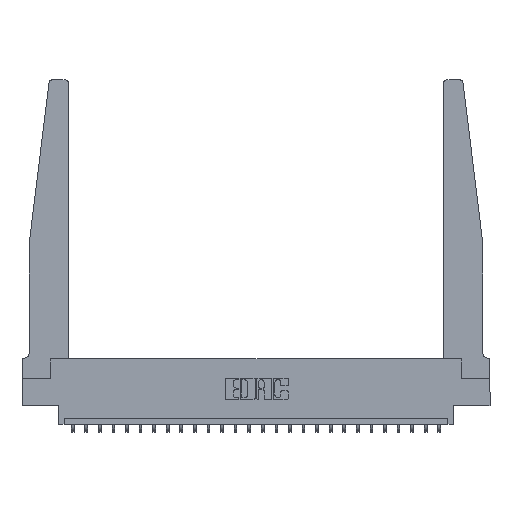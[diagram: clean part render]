
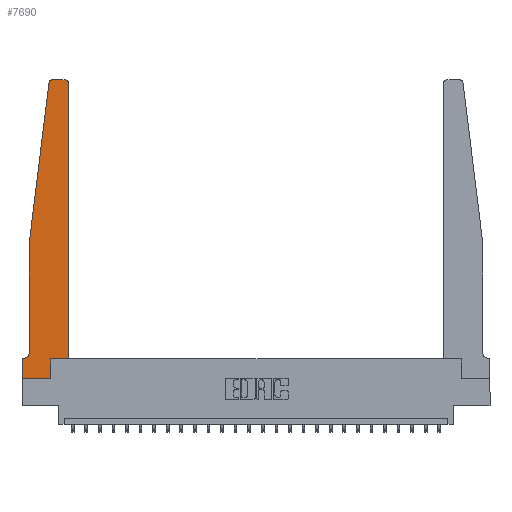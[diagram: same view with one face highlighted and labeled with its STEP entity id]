
A CAD part, top view. The second image highlights one B-rep face of the part: STEP entity #7690.
In plain terms, the highlighted planar face has unit normal (0, 0, 1).
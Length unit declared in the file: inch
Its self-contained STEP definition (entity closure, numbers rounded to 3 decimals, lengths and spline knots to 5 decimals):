
#848 = CIRCLE ( 'NONE', #6700, 0.03 ) ;
#877 = DIRECTION ( 'NONE',  ( 0., -1., 0. ) ) ;
#1224 = CARTESIAN_POINT ( 'NONE',  ( 0.065, 0.2375, 0.37 ) ) ;
#1806 = DIRECTION ( 'NONE',  ( 1., 0., 0. ) ) ;
#1873 = VERTEX_POINT ( 'NONE', #12678 ) ;
#2963 = ORIENTED_EDGE ( 'NONE', *, *, #17596, .T. ) ;
#3009 = VECTOR ( 'NONE', #11508, 39.37008 ) ;
#3305 = EDGE_CURVE ( 'NONE', #21241, #8858, #13547, .T. ) ;
#3498 = LINE ( 'NONE', #13590, #21638 ) ;
#3528 = CARTESIAN_POINT ( 'NONE',  ( 0.395, 2.72, 0.37 ) ) ;
#3732 = CARTESIAN_POINT ( 'NONE',  ( 0.065, 0.1875, 0.37 ) ) ;
#4224 = DIRECTION ( 'NONE',  ( -0.122, -0.992, 0. ) ) ;
#4286 = CARTESIAN_POINT ( 'NONE',  ( 0.2605, 0., 0.37 ) ) ;
#4564 = EDGE_CURVE ( 'NONE', #17738, #1873, #848, .T. ) ;
#4660 = VERTEX_POINT ( 'NONE', #21850 ) ;
#4731 = EDGE_CURVE ( 'NONE', #16725, #4660, #22803, .T. ) ;
#5137 = LINE ( 'NONE', #17966, #23874 ) ;
#5405 = DIRECTION ( 'NONE',  ( 1., 0., 0. ) ) ;
#5540 = VERTEX_POINT ( 'NONE', #5932 ) ;
#5932 = CARTESIAN_POINT ( 'NONE',  ( 0.395, 2.75, 0.37 ) ) ;
#5989 = VERTEX_POINT ( 'NONE', #16567 ) ;
#6015 = CARTESIAN_POINT ( 'NONE',  ( 0., 0., 0.37 ) ) ;
#6136 = DIRECTION ( 'NONE',  ( 1., 0., 0. ) ) ;
#6283 = ORIENTED_EDGE ( 'NONE', *, *, #21321, .T. ) ;
#6534 = VECTOR ( 'NONE', #1806, 39.37008 ) ;
#6631 = CARTESIAN_POINT ( 'NONE',  ( 0.27653, 2.75, 0.37 ) ) ;
#6700 = AXIS2_PLACEMENT_3D ( 'NONE', #10417, #23488, #12304 ) ;
#6841 = EDGE_CURVE ( 'NONE', #10985, #21241, #22988, .T. ) ;
#6980 = EDGE_CURVE ( 'NONE', #5540, #17738, #5137, .T. ) ;
#7046 = EDGE_LOOP ( 'NONE', ( #7578, #17709, #7866, #20436, #24205, #12894, #13224, #21968, #2963, #16415, #7968, #6283 ) ) ;
#7367 = CARTESIAN_POINT ( 'NONE',  ( 0.2605, 0.18, 0.37 ) ) ;
#7578 = ORIENTED_EDGE ( 'NONE', *, *, #6980, .T. ) ;
#7690 = ADVANCED_FACE ( 'NONE', ( #17716 ), #15469, .T. ) ;
#7740 = CARTESIAN_POINT ( 'NONE',  ( 0., 0., 0.37 ) ) ;
#7866 = ORIENTED_EDGE ( 'NONE', *, *, #9949, .T. ) ;
#7924 = DIRECTION ( 'NONE',  ( 1., 0., 0. ) ) ;
#7968 = ORIENTED_EDGE ( 'NONE', *, *, #4731, .T. ) ;
#8472 = LINE ( 'NONE', #6015, #17218 ) ;
#8858 = VERTEX_POINT ( 'NONE', #15163 ) ;
#9049 = CARTESIAN_POINT ( 'NONE',  ( 0.425, 0.18, 0.37 ) ) ;
#9165 = CIRCLE ( 'NONE', #15791, 0.03 ) ;
#9415 = VECTOR ( 'NONE', #11869, 39.37008 ) ;
#9768 = EDGE_CURVE ( 'NONE', #8858, #17679, #10851, .T. ) ;
#9903 = DIRECTION ( 'NONE',  ( 0., 0., -1. ) ) ;
#9949 = EDGE_CURVE ( 'NONE', #1873, #10985, #3498, .T. ) ;
#10417 = CARTESIAN_POINT ( 'NONE',  ( 0.27653, 2.72, 0.37 ) ) ;
#10851 = LINE ( 'NONE', #3732, #15813 ) ;
#10917 = CARTESIAN_POINT ( 'NONE',  ( 0.425, 0.18, 0.37 ) ) ;
#10985 = VERTEX_POINT ( 'NONE', #12646 ) ;
#11508 = DIRECTION ( 'NONE',  ( 0., -1., 0. ) ) ;
#11869 = DIRECTION ( 'NONE',  ( 0., 1., 0. ) ) ;
#12304 = DIRECTION ( 'NONE',  ( 1., 0., 0. ) ) ;
#12646 = CARTESIAN_POINT ( 'NONE',  ( 0.065, 1.25, 0.37 ) ) ;
#12678 = CARTESIAN_POINT ( 'NONE',  ( 0.24675, 2.72367, 0.37 ) ) ;
#12894 = ORIENTED_EDGE ( 'NONE', *, *, #9768, .T. ) ;
#13064 = CARTESIAN_POINT ( 'NONE',  ( 0.425, 0.18, 0.37 ) ) ;
#13224 = ORIENTED_EDGE ( 'NONE', *, *, #20869, .T. ) ;
#13547 = CIRCLE ( 'NONE', #21059, 0.05 ) ;
#13590 = CARTESIAN_POINT ( 'NONE',  ( 0.065, 1.25, 0.37 ) ) ;
#13686 = VERTEX_POINT ( 'NONE', #4286 ) ;
#13914 = CARTESIAN_POINT ( 'NONE',  ( 0., 0.1875, 0.37 ) ) ;
#13995 = CARTESIAN_POINT ( 'NONE',  ( 0.065, 1.25, 0.37 ) ) ;
#14399 = LINE ( 'NONE', #23038, #9415 ) ;
#14655 = VERTEX_POINT ( 'NONE', #7367 ) ;
#15163 = CARTESIAN_POINT ( 'NONE',  ( 0.015, 0.1875, 0.37 ) ) ;
#15469 = PLANE ( 'NONE',  #22471 ) ;
#15791 = AXIS2_PLACEMENT_3D ( 'NONE', #3528, #16635, #5405 ) ;
#15813 = VECTOR ( 'NONE', #16824, 39.37008 ) ;
#16415 = ORIENTED_EDGE ( 'NONE', *, *, #16810, .T. ) ;
#16567 = CARTESIAN_POINT ( 'NONE',  ( 0., 0., 0.37 ) ) ;
#16635 = DIRECTION ( 'NONE',  ( 0., 0., 1. ) ) ;
#16725 = VERTEX_POINT ( 'NONE', #9049 ) ;
#16810 = EDGE_CURVE ( 'NONE', #14655, #16725, #21431, .T. ) ;
#16824 = DIRECTION ( 'NONE',  ( -1., 0., 0. ) ) ;
#17218 = VECTOR ( 'NONE', #7924, 39.37008 ) ;
#17338 = DIRECTION ( 'NONE',  ( 0., 0., 1. ) ) ;
#17596 = EDGE_CURVE ( 'NONE', #13686, #14655, #14399, .T. ) ;
#17679 = VERTEX_POINT ( 'NONE', #13914 ) ;
#17709 = ORIENTED_EDGE ( 'NONE', *, *, #4564, .T. ) ;
#17716 = FACE_OUTER_BOUND ( 'NONE', #7046, .T. ) ;
#17738 = VERTEX_POINT ( 'NONE', #6631 ) ;
#17926 = LINE ( 'NONE', #7740, #3009 ) ;
#17966 = CARTESIAN_POINT ( 'NONE',  ( 0.25, 2.75, 0.37 ) ) ;
#19358 = EDGE_CURVE ( 'NONE', #5989, #13686, #8472, .T. ) ;
#20436 = ORIENTED_EDGE ( 'NONE', *, *, #6841, .T. ) ;
#20869 = EDGE_CURVE ( 'NONE', #17679, #5989, #17926, .T. ) ;
#21059 = AXIS2_PLACEMENT_3D ( 'NONE', #21077, #9903, #22953 ) ;
#21077 = CARTESIAN_POINT ( 'NONE',  ( 0.015, 0.2375, 0.37 ) ) ;
#21241 = VERTEX_POINT ( 'NONE', #1224 ) ;
#21321 = EDGE_CURVE ( 'NONE', #4660, #5540, #9165, .T. ) ;
#21431 = LINE ( 'NONE', #13064, #6534 ) ;
#21632 = VECTOR ( 'NONE', #22101, 39.37008 ) ;
#21638 = VECTOR ( 'NONE', #4224, 39.37008 ) ;
#21850 = CARTESIAN_POINT ( 'NONE',  ( 0.425, 2.72, 0.37 ) ) ;
#21968 = ORIENTED_EDGE ( 'NONE', *, *, #19358, .T. ) ;
#22101 = DIRECTION ( 'NONE',  ( 0., 1., 0. ) ) ;
#22471 = AXIS2_PLACEMENT_3D ( 'NONE', #22885, #17338, #6136 ) ;
#22803 = LINE ( 'NONE', #10917, #21632 ) ;
#22885 = CARTESIAN_POINT ( 'NONE',  ( 0., 0.1875, 0.37 ) ) ;
#22953 = DIRECTION ( 'NONE',  ( -1., 0., 0. ) ) ;
#22988 = LINE ( 'NONE', #13995, #23588 ) ;
#23038 = CARTESIAN_POINT ( 'NONE',  ( 0.2605, 0.18, 0.37 ) ) ;
#23488 = DIRECTION ( 'NONE',  ( 0., 0., 1. ) ) ;
#23588 = VECTOR ( 'NONE', #877, 39.37008 ) ;
#23621 = DIRECTION ( 'NONE',  ( -1., 0., 0. ) ) ;
#23874 = VECTOR ( 'NONE', #23621, 39.37008 ) ;
#24205 = ORIENTED_EDGE ( 'NONE', *, *, #3305, .T. ) ;
